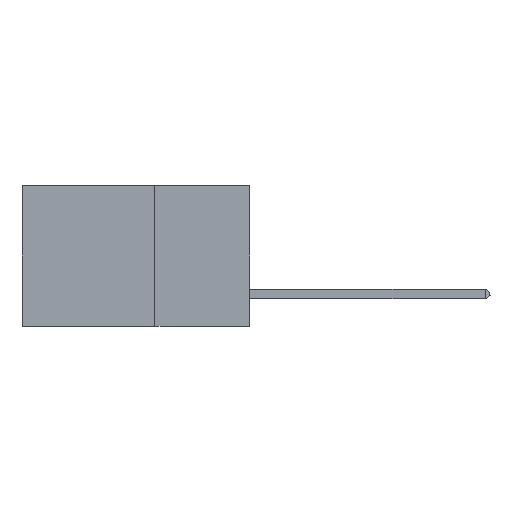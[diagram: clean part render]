
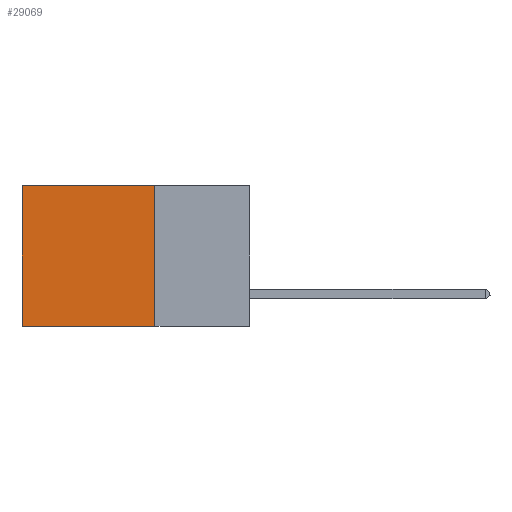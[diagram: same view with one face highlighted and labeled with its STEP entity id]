
A CAD part, left-side view. The second image highlights one B-rep face of the part: STEP entity #29069.
In plain terms, the highlighted planar face has unit normal (-1, 0, 0).
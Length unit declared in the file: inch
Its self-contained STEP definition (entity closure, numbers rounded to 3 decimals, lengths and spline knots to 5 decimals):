
#54 = CARTESIAN_POINT ( 'NONE',  ( 0.2875, 0.25, 0. ) ) ;
#1417 = CARTESIAN_POINT ( 'NONE',  ( 0.2875, 0.6, 0. ) ) ;
#2347 = VERTEX_POINT ( 'NONE', #30857 ) ;
#2531 = CARTESIAN_POINT ( 'NONE',  ( 0.2875, 0.25, 0. ) ) ;
#2583 = ORIENTED_EDGE ( 'NONE', *, *, #7308, .F. ) ;
#2776 = VERTEX_POINT ( 'NONE', #4304 ) ;
#3706 = ORIENTED_EDGE ( 'NONE', *, *, #9534, .F. ) ;
#4053 = EDGE_CURVE ( 'NONE', #8894, #2347, #14591, .T. ) ;
#4304 = CARTESIAN_POINT ( 'NONE',  ( 0.2875, 0.25, -0.37 ) ) ;
#4464 = EDGE_LOOP ( 'NONE', ( #7782, #3706, #2583, #18911 ) ) ;
#5217 = DIRECTION ( 'NONE',  ( 0., 0., -1. ) ) ;
#5307 = DIRECTION ( 'NONE',  ( 0., 1., 0. ) ) ;
#5606 = CARTESIAN_POINT ( 'NONE',  ( 0.2875, 0.25, -0.37 ) ) ;
#7308 = EDGE_CURVE ( 'NONE', #8894, #2776, #14168, .T. ) ;
#7782 = ORIENTED_EDGE ( 'NONE', *, *, #12076, .T. ) ;
#8500 = CARTESIAN_POINT ( 'NONE',  ( 0.2875, 0.25, 0. ) ) ;
#8648 = DIRECTION ( 'NONE',  ( 0., 0., -1. ) ) ;
#8894 = VERTEX_POINT ( 'NONE', #30619 ) ;
#9534 = EDGE_CURVE ( 'NONE', #2776, #20257, #25685, .T. ) ;
#11961 = AXIS2_PLACEMENT_3D ( 'NONE', #2531, #19526, #5217 ) ;
#12030 = VECTOR ( 'NONE', #30552, 39.37008 ) ;
#12076 = EDGE_CURVE ( 'NONE', #2347, #20257, #23676, .T. ) ;
#12089 = VECTOR ( 'NONE', #8648, 39.37008 ) ;
#12624 = VECTOR ( 'NONE', #26093, 39.37008 ) ;
#14168 = LINE ( 'NONE', #54, #12624 ) ;
#14591 = LINE ( 'NONE', #8500, #12030 ) ;
#14623 = PLANE ( 'NONE',  #11961 ) ;
#17065 = CARTESIAN_POINT ( 'NONE',  ( 0.2875, 0.6, -0.37 ) ) ;
#18911 = ORIENTED_EDGE ( 'NONE', *, *, #4053, .T. ) ;
#19526 = DIRECTION ( 'NONE',  ( 1., 0., 0. ) ) ;
#20257 = VERTEX_POINT ( 'NONE', #17065 ) ;
#21293 = FACE_OUTER_BOUND ( 'NONE', #4464, .T. ) ;
#23028 = VECTOR ( 'NONE', #5307, 39.37008 ) ;
#23676 = LINE ( 'NONE', #1417, #12089 ) ;
#25685 = LINE ( 'NONE', #5606, #23028 ) ;
#26093 = DIRECTION ( 'NONE',  ( 0., 0., -1. ) ) ;
#29069 = ADVANCED_FACE ( 'NONE', ( #21293 ), #14623, .F. ) ;
#30552 = DIRECTION ( 'NONE',  ( 0., 1., 0. ) ) ;
#30619 = CARTESIAN_POINT ( 'NONE',  ( 0.2875, 0.25, 0. ) ) ;
#30857 = CARTESIAN_POINT ( 'NONE',  ( 0.2875, 0.6, 0. ) ) ;
